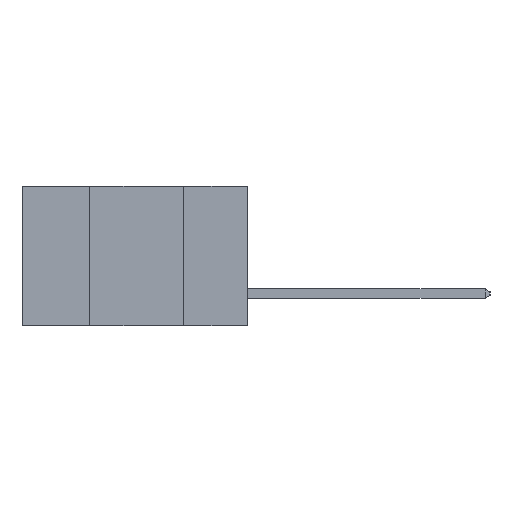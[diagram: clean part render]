
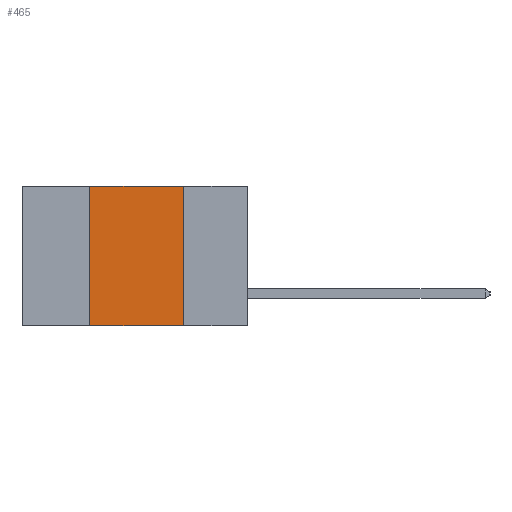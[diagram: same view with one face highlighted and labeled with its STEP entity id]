
A CAD part, left-side view. The second image highlights one B-rep face of the part: STEP entity #465.
In plain terms, the highlighted planar face has unit normal (-1, 0, 0).
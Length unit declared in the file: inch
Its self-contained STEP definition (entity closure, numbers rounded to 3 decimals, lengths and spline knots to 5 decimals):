
#465 = ADVANCED_FACE ( 'NONE', ( #8045 ), #9120, .F. ) ;
#656 = VERTEX_POINT ( 'NONE', #5449 ) ;
#853 = DIRECTION ( 'NONE',  ( 0., -1., 0. ) ) ;
#970 = VECTOR ( 'NONE', #853, 39.37008 ) ;
#1057 = CARTESIAN_POINT ( 'NONE',  ( 0., 0.42, -0.37 ) ) ;
#1195 = VECTOR ( 'NONE', #10887, 39.37008 ) ;
#1967 = VERTEX_POINT ( 'NONE', #1057 ) ;
#1981 = VECTOR ( 'NONE', #2599, 39.37008 ) ;
#2171 = AXIS2_PLACEMENT_3D ( 'NONE', #6322, #10520, #2408 ) ;
#2408 = DIRECTION ( 'NONE',  ( 0., 0., -1. ) ) ;
#2573 = VERTEX_POINT ( 'NONE', #3280 ) ;
#2599 = DIRECTION ( 'NONE',  ( 0., 0., 1. ) ) ;
#2869 = DIRECTION ( 'NONE',  ( 0., -1., 0. ) ) ;
#2932 = CARTESIAN_POINT ( 'NONE',  ( 0., 0.6, 0. ) ) ;
#3007 = CARTESIAN_POINT ( 'NONE',  ( 0., 0.17, -0.37 ) ) ;
#3178 = ORIENTED_EDGE ( 'NONE', *, *, #4207, .F. ) ;
#3280 = CARTESIAN_POINT ( 'NONE',  ( 0., 0.17, -0.37 ) ) ;
#3332 = LINE ( 'NONE', #3007, #1195 ) ;
#3406 = LINE ( 'NONE', #8671, #970 ) ;
#3728 = EDGE_CURVE ( 'NONE', #6902, #656, #8186, .T. ) ;
#4207 = EDGE_CURVE ( 'NONE', #656, #2573, #3332, .T. ) ;
#4705 = ORIENTED_EDGE ( 'NONE', *, *, #9226, .T. ) ;
#5449 = CARTESIAN_POINT ( 'NONE',  ( 0., 0.17, 0. ) ) ;
#6322 = CARTESIAN_POINT ( 'NONE',  ( 0., 0.6, 0. ) ) ;
#6410 = EDGE_LOOP ( 'NONE', ( #3178, #9377, #7860, #4705 ) ) ;
#6681 = LINE ( 'NONE', #8598, #1981 ) ;
#6902 = VERTEX_POINT ( 'NONE', #11033 ) ;
#7860 = ORIENTED_EDGE ( 'NONE', *, *, #9761, .F. ) ;
#8045 = FACE_OUTER_BOUND ( 'NONE', #6410, .T. ) ;
#8186 = LINE ( 'NONE', #2932, #10066 ) ;
#8598 = CARTESIAN_POINT ( 'NONE',  ( 0., 0.42, -0.37 ) ) ;
#8671 = CARTESIAN_POINT ( 'NONE',  ( 0., 0.6, -0.37 ) ) ;
#9120 = PLANE ( 'NONE',  #2171 ) ;
#9226 = EDGE_CURVE ( 'NONE', #1967, #2573, #3406, .T. ) ;
#9377 = ORIENTED_EDGE ( 'NONE', *, *, #3728, .F. ) ;
#9761 = EDGE_CURVE ( 'NONE', #1967, #6902, #6681, .T. ) ;
#10066 = VECTOR ( 'NONE', #2869, 39.37008 ) ;
#10520 = DIRECTION ( 'NONE',  ( 1., 0., 0. ) ) ;
#10887 = DIRECTION ( 'NONE',  ( 0., 0., -1. ) ) ;
#11033 = CARTESIAN_POINT ( 'NONE',  ( 0., 0.42, 0. ) ) ;
